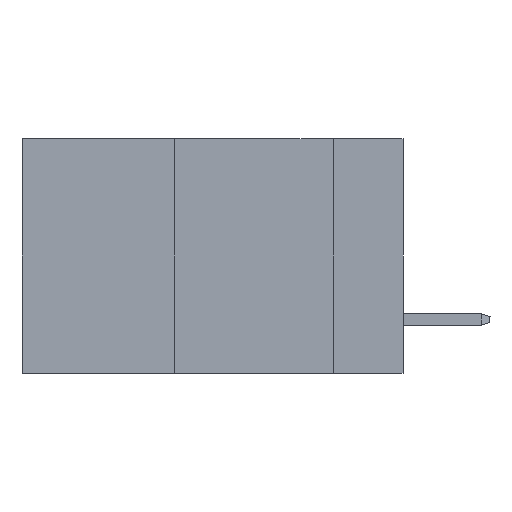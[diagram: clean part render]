
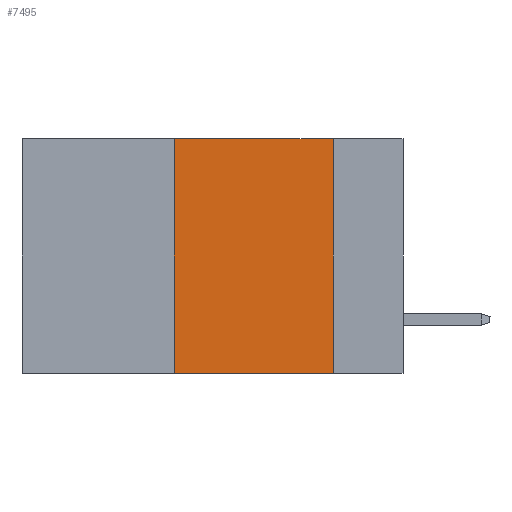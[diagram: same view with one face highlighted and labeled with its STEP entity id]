
A CAD part, left-side view. The second image highlights one B-rep face of the part: STEP entity #7495.
In plain terms, the highlighted planar face has unit normal (-1, 0, 0).
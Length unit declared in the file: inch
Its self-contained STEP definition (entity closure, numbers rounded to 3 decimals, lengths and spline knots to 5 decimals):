
#254 = DIRECTION ( 'NONE',  ( 0., -1., 0. ) ) ;
#894 = CARTESIAN_POINT ( 'NONE',  ( 0., 0.36, -0.37 ) ) ;
#1293 = CARTESIAN_POINT ( 'NONE',  ( 0., 0.11, -0.37 ) ) ;
#1914 = ORIENTED_EDGE ( 'NONE', *, *, #5208, .F. ) ;
#3424 = VECTOR ( 'NONE', #254, 39.37008 ) ;
#3526 = EDGE_CURVE ( 'NONE', #9705, #21930, #23268, .T. ) ;
#3582 = DIRECTION ( 'NONE',  ( 0., 0., 1. ) ) ;
#5208 = EDGE_CURVE ( 'NONE', #9705, #23617, #16698, .T. ) ;
#6335 = CARTESIAN_POINT ( 'NONE',  ( 0., 0.11, 0. ) ) ;
#6498 = FACE_OUTER_BOUND ( 'NONE', #19318, .T. ) ;
#6937 = EDGE_CURVE ( 'NONE', #23521, #21930, #24552, .T. ) ;
#7495 = ADVANCED_FACE ( 'NONE', ( #6498 ), #16036, .F. ) ;
#9705 = VERTEX_POINT ( 'NONE', #894 ) ;
#10030 = AXIS2_PLACEMENT_3D ( 'NONE', #14134, #14258, #12333 ) ;
#12333 = DIRECTION ( 'NONE',  ( 0., 0., -1. ) ) ;
#13068 = ORIENTED_EDGE ( 'NONE', *, *, #6937, .F. ) ;
#14027 = EDGE_CURVE ( 'NONE', #23617, #23521, #16316, .T. ) ;
#14134 = CARTESIAN_POINT ( 'NONE',  ( 0., 0.6, 0. ) ) ;
#14258 = DIRECTION ( 'NONE',  ( 1., 0., 0. ) ) ;
#16036 = PLANE ( 'NONE',  #10030 ) ;
#16057 = VECTOR ( 'NONE', #3582, 39.37008 ) ;
#16316 = LINE ( 'NONE', #18194, #17835 ) ;
#16698 = LINE ( 'NONE', #22594, #16057 ) ;
#16865 = CARTESIAN_POINT ( 'NONE',  ( 0., 0.36, 0. ) ) ;
#17299 = VECTOR ( 'NONE', #22505, 39.37008 ) ;
#17835 = VECTOR ( 'NONE', #20099, 39.37008 ) ;
#18194 = CARTESIAN_POINT ( 'NONE',  ( 0., 0.6, 0. ) ) ;
#19318 = EDGE_LOOP ( 'NONE', ( #13068, #22143, #1914, #23692 ) ) ;
#20099 = DIRECTION ( 'NONE',  ( 0., -1., 0. ) ) ;
#21930 = VERTEX_POINT ( 'NONE', #1293 ) ;
#22143 = ORIENTED_EDGE ( 'NONE', *, *, #14027, .F. ) ;
#22505 = DIRECTION ( 'NONE',  ( 0., 0., -1. ) ) ;
#22594 = CARTESIAN_POINT ( 'NONE',  ( 0., 0.36, 0. ) ) ;
#22635 = CARTESIAN_POINT ( 'NONE',  ( 0., 0.11, 0. ) ) ;
#22789 = CARTESIAN_POINT ( 'NONE',  ( 0., 0.6, -0.37 ) ) ;
#23268 = LINE ( 'NONE', #22789, #3424 ) ;
#23521 = VERTEX_POINT ( 'NONE', #6335 ) ;
#23617 = VERTEX_POINT ( 'NONE', #16865 ) ;
#23692 = ORIENTED_EDGE ( 'NONE', *, *, #3526, .T. ) ;
#24552 = LINE ( 'NONE', #22635, #17299 ) ;
